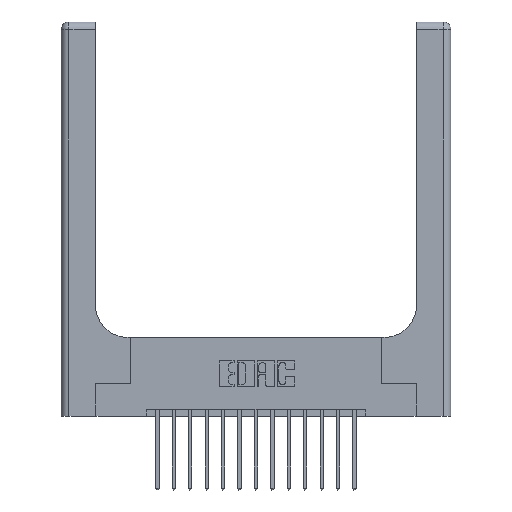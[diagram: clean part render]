
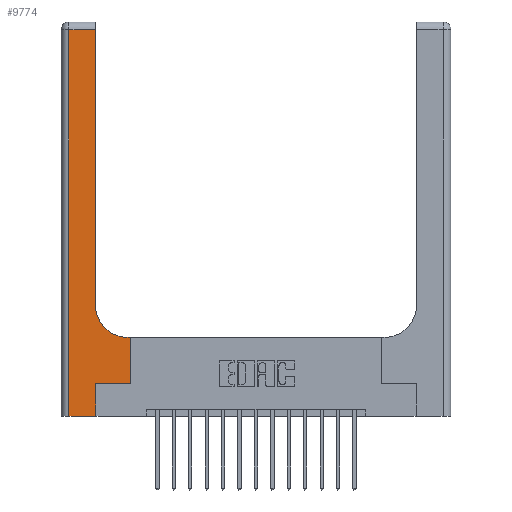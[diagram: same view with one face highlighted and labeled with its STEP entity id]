
A CAD part, top view. The second image highlights one B-rep face of the part: STEP entity #9774.
In plain terms, the highlighted planar face has unit normal (0, 0, 1).
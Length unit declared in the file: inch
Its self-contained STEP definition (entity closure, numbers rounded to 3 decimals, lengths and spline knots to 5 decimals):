
#264 = LINE ( 'NONE', #12958, #1841 ) ;
#284 = CARTESIAN_POINT ( 'NONE',  ( 0.26, 0.6, 0.37 ) ) ;
#651 = VERTEX_POINT ( 'NONE', #15493 ) ;
#674 = EDGE_LOOP ( 'NONE', ( #1523, #6695, #8096, #5260, #2512, #15565, #10149, #5501, #14904 ) ) ;
#697 = DIRECTION ( 'NONE',  ( -1., 0., 0. ) ) ;
#992 = VERTEX_POINT ( 'NONE', #4276 ) ;
#1126 = EDGE_CURVE ( 'NONE', #5095, #1650, #13048, .T. ) ;
#1523 = ORIENTED_EDGE ( 'NONE', *, *, #1126, .T. ) ;
#1650 = VERTEX_POINT ( 'NONE', #10996 ) ;
#1841 = VECTOR ( 'NONE', #7128, 39.37008 ) ;
#2056 = DIRECTION ( 'NONE',  ( 0., 1., 0. ) ) ;
#2390 = CARTESIAN_POINT ( 'NONE',  ( 0.51, 0.85, 0.37 ) ) ;
#2498 = DIRECTION ( 'NONE',  ( 1., 0., 0. ) ) ;
#2512 = ORIENTED_EDGE ( 'NONE', *, *, #16095, .T. ) ;
#2560 = AXIS2_PLACEMENT_3D ( 'NONE', #6889, #9620, #14836 ) ;
#4276 = CARTESIAN_POINT ( 'NONE',  ( 0.528, 0.6, 0.37 ) ) ;
#4351 = VERTEX_POINT ( 'NONE', #14931 ) ;
#4811 = LINE ( 'NONE', #13228, #16863 ) ;
#5095 = VERTEX_POINT ( 'NONE', #5254 ) ;
#5254 = CARTESIAN_POINT ( 'NONE',  ( 0.26, 0.85, 0.37 ) ) ;
#5260 = ORIENTED_EDGE ( 'NONE', *, *, #7406, .T. ) ;
#5501 = ORIENTED_EDGE ( 'NONE', *, *, #17484, .T. ) ;
#5859 = DIRECTION ( 'NONE',  ( -1., 0., 0. ) ) ;
#5953 = CIRCLE ( 'NONE', #10025, 0.25 ) ;
#6123 = CARTESIAN_POINT ( 'NONE',  ( 0.26, 3., 0.37 ) ) ;
#6206 = EDGE_CURVE ( 'NONE', #1650, #9476, #4811, .T. ) ;
#6695 = ORIENTED_EDGE ( 'NONE', *, *, #6206, .T. ) ;
#6781 = CARTESIAN_POINT ( 'NONE',  ( 0.06, 3., 0.37 ) ) ;
#6889 = CARTESIAN_POINT ( 'NONE',  ( 0., 3., 0.37 ) ) ;
#6911 = CARTESIAN_POINT ( 'NONE',  ( 0.265, 0.25, 0.37 ) ) ;
#7037 = CARTESIAN_POINT ( 'NONE',  ( 0.528, 0.25, 0.37 ) ) ;
#7128 = DIRECTION ( 'NONE',  ( 0., 1., 0. ) ) ;
#7406 = EDGE_CURVE ( 'NONE', #15901, #651, #8678, .T. ) ;
#7851 = CARTESIAN_POINT ( 'NONE',  ( 0.06, 0., 0.37 ) ) ;
#7877 = DIRECTION ( 'NONE',  ( 1., 0., 0. ) ) ;
#7910 = VERTEX_POINT ( 'NONE', #11743 ) ;
#8096 = ORIENTED_EDGE ( 'NONE', *, *, #12113, .T. ) ;
#8577 = CARTESIAN_POINT ( 'NONE',  ( 0., 0., 0.37 ) ) ;
#8678 = LINE ( 'NONE', #8577, #12856 ) ;
#9476 = VERTEX_POINT ( 'NONE', #13581 ) ;
#9620 = DIRECTION ( 'NONE',  ( 0., 0., -1. ) ) ;
#9690 = DIRECTION ( 'NONE',  ( 0., 1., 0. ) ) ;
#9774 = ADVANCED_FACE ( 'NONE', ( #17908 ), #15014, .F. ) ;
#10025 = AXIS2_PLACEMENT_3D ( 'NONE', #2390, #14845, #7877 ) ;
#10086 = EDGE_CURVE ( 'NONE', #4351, #13785, #13865, .T. ) ;
#10149 = ORIENTED_EDGE ( 'NONE', *, *, #17776, .T. ) ;
#10624 = VECTOR ( 'NONE', #2056, 39.37008 ) ;
#10996 = CARTESIAN_POINT ( 'NONE',  ( 0.26, 2.94, 0.37 ) ) ;
#11743 = CARTESIAN_POINT ( 'NONE',  ( 0.51, 0.6, 0.37 ) ) ;
#12113 = EDGE_CURVE ( 'NONE', #9476, #15901, #15284, .T. ) ;
#12430 = CARTESIAN_POINT ( 'NONE',  ( 0.265, 0., 0.37 ) ) ;
#12487 = VECTOR ( 'NONE', #2498, 39.37008 ) ;
#12778 = DIRECTION ( 'NONE',  ( 1., 0., 0. ) ) ;
#12798 = LINE ( 'NONE', #284, #14983 ) ;
#12856 = VECTOR ( 'NONE', #12778, 39.37008 ) ;
#12958 = CARTESIAN_POINT ( 'NONE',  ( 0.528, 0.25, 0.37 ) ) ;
#13048 = LINE ( 'NONE', #6123, #10624 ) ;
#13228 = CARTESIAN_POINT ( 'NONE',  ( 0., 2.94, 0.37 ) ) ;
#13581 = CARTESIAN_POINT ( 'NONE',  ( 0.06, 2.94, 0.37 ) ) ;
#13785 = VERTEX_POINT ( 'NONE', #7037 ) ;
#13865 = LINE ( 'NONE', #6911, #12487 ) ;
#14836 = DIRECTION ( 'NONE',  ( -1., 0., 0. ) ) ;
#14845 = DIRECTION ( 'NONE',  ( 0., 0., -1. ) ) ;
#14904 = ORIENTED_EDGE ( 'NONE', *, *, #17341, .T. ) ;
#14931 = CARTESIAN_POINT ( 'NONE',  ( 0.265, 0.25, 0.37 ) ) ;
#14983 = VECTOR ( 'NONE', #5859, 39.37008 ) ;
#14999 = DIRECTION ( 'NONE',  ( 0., -1., 0. ) ) ;
#15014 = PLANE ( 'NONE',  #2560 ) ;
#15284 = LINE ( 'NONE', #6781, #15782 ) ;
#15493 = CARTESIAN_POINT ( 'NONE',  ( 0.265, 0., 0.37 ) ) ;
#15565 = ORIENTED_EDGE ( 'NONE', *, *, #10086, .T. ) ;
#15585 = VECTOR ( 'NONE', #9690, 39.37008 ) ;
#15782 = VECTOR ( 'NONE', #14999, 39.37008 ) ;
#15901 = VERTEX_POINT ( 'NONE', #7851 ) ;
#16095 = EDGE_CURVE ( 'NONE', #651, #4351, #16633, .T. ) ;
#16633 = LINE ( 'NONE', #12430, #15585 ) ;
#16863 = VECTOR ( 'NONE', #697, 39.37008 ) ;
#17341 = EDGE_CURVE ( 'NONE', #7910, #5095, #5953, .T. ) ;
#17484 = EDGE_CURVE ( 'NONE', #992, #7910, #12798, .T. ) ;
#17776 = EDGE_CURVE ( 'NONE', #13785, #992, #264, .T. ) ;
#17908 = FACE_OUTER_BOUND ( 'NONE', #674, .T. ) ;
